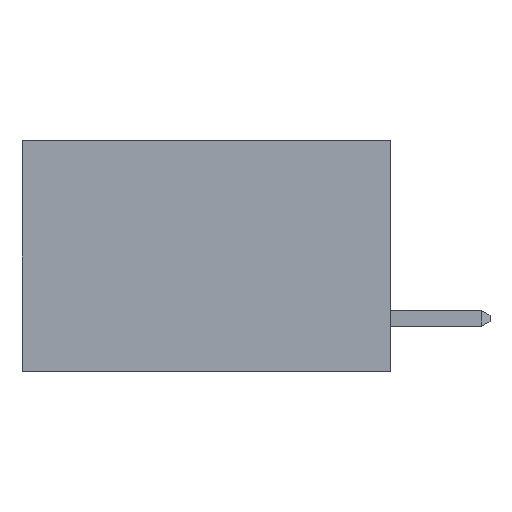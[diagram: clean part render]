
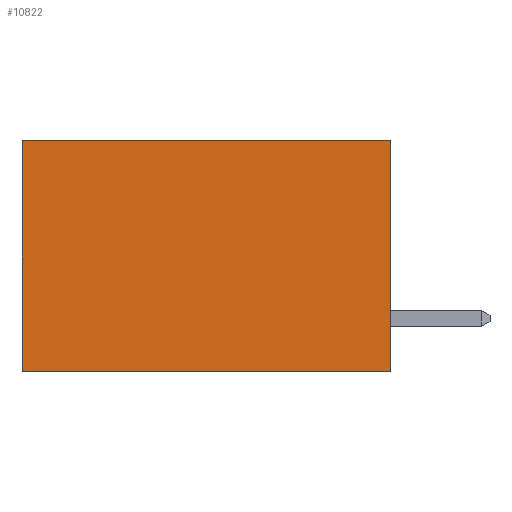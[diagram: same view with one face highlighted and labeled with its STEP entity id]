
A CAD part, left-side view. The second image highlights one B-rep face of the part: STEP entity #10822.
In plain terms, the highlighted planar face has unit normal (-1, 0, 0).
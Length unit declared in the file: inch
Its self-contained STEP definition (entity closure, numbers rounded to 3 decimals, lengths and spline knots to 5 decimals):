
#1126 = CARTESIAN_POINT ( 'NONE',  ( 0.277, 0., -0.37 ) ) ;
#1427 = CARTESIAN_POINT ( 'NONE',  ( 0.277, 0.59, 0. ) ) ;
#1485 = CARTESIAN_POINT ( 'NONE',  ( 0.277, 0.59, -0.37 ) ) ;
#2400 = EDGE_LOOP ( 'NONE', ( #9990, #18667, #20359, #20963 ) ) ;
#2904 = DIRECTION ( 'NONE',  ( 0., 0., -1. ) ) ;
#3112 = DIRECTION ( 'NONE',  ( 0., 0., -1. ) ) ;
#3371 = LINE ( 'NONE', #17697, #5639 ) ;
#3931 = CARTESIAN_POINT ( 'NONE',  ( 0.277, 0.59, -0.37 ) ) ;
#4492 = AXIS2_PLACEMENT_3D ( 'NONE', #19024, #12601, #2904 ) ;
#4819 = DIRECTION ( 'NONE',  ( 0., 0., -1. ) ) ;
#5639 = VECTOR ( 'NONE', #19251, 39.37008 ) ;
#6018 = CARTESIAN_POINT ( 'NONE',  ( 0.277, 0., -0.37 ) ) ;
#6117 = VERTEX_POINT ( 'NONE', #1126 ) ;
#7259 = VERTEX_POINT ( 'NONE', #15024 ) ;
#9549 = LINE ( 'NONE', #6018, #13390 ) ;
#9914 = LINE ( 'NONE', #12898, #13753 ) ;
#9990 = ORIENTED_EDGE ( 'NONE', *, *, #12280, .T. ) ;
#10765 = EDGE_CURVE ( 'NONE', #6117, #17433, #9549, .T. ) ;
#10822 = ADVANCED_FACE ( 'NONE', ( #16684 ), #20615, .F. ) ;
#12280 = EDGE_CURVE ( 'NONE', #19214, #17433, #16376, .T. ) ;
#12601 = DIRECTION ( 'NONE',  ( 1., 0., 0. ) ) ;
#12898 = CARTESIAN_POINT ( 'NONE',  ( 0.277, 0., -0.37 ) ) ;
#13390 = VECTOR ( 'NONE', #18962, 39.37008 ) ;
#13682 = EDGE_CURVE ( 'NONE', #7259, #19214, #3371, .T. ) ;
#13697 = EDGE_CURVE ( 'NONE', #7259, #6117, #9914, .T. ) ;
#13753 = VECTOR ( 'NONE', #4819, 39.37008 ) ;
#15024 = CARTESIAN_POINT ( 'NONE',  ( 0.277, 0., 0. ) ) ;
#16376 = LINE ( 'NONE', #1485, #20098 ) ;
#16684 = FACE_OUTER_BOUND ( 'NONE', #2400, .T. ) ;
#17433 = VERTEX_POINT ( 'NONE', #3931 ) ;
#17697 = CARTESIAN_POINT ( 'NONE',  ( 0.277, 0., 0. ) ) ;
#18667 = ORIENTED_EDGE ( 'NONE', *, *, #10765, .F. ) ;
#18962 = DIRECTION ( 'NONE',  ( 0., 1., 0. ) ) ;
#19024 = CARTESIAN_POINT ( 'NONE',  ( 0.277, 0., -0.37 ) ) ;
#19214 = VERTEX_POINT ( 'NONE', #1427 ) ;
#19251 = DIRECTION ( 'NONE',  ( 0., 1., 0. ) ) ;
#20098 = VECTOR ( 'NONE', #3112, 39.37008 ) ;
#20359 = ORIENTED_EDGE ( 'NONE', *, *, #13697, .F. ) ;
#20615 = PLANE ( 'NONE',  #4492 ) ;
#20963 = ORIENTED_EDGE ( 'NONE', *, *, #13682, .T. ) ;
